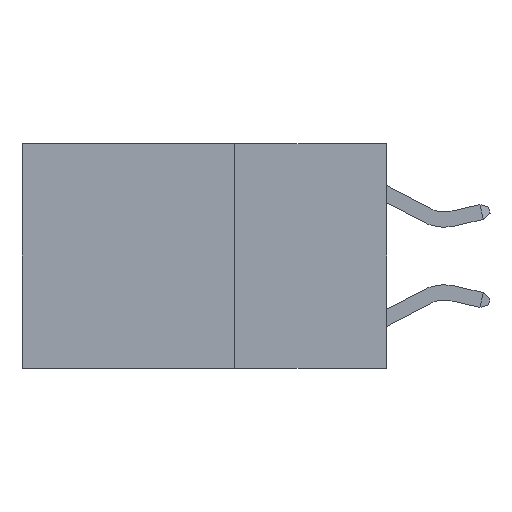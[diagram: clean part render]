
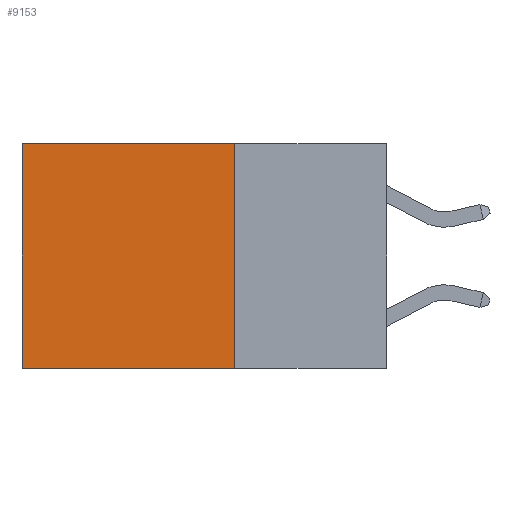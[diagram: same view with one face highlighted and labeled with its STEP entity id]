
A CAD part, left-side view. The second image highlights one B-rep face of the part: STEP entity #9153.
In plain terms, the highlighted planar face has unit normal (-1, 0, 0).
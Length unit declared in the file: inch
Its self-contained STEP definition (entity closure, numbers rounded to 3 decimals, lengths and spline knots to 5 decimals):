
#98 = VERTEX_POINT ( 'NONE', #7601 ) ;
#536 = VERTEX_POINT ( 'NONE', #4608 ) ;
#1321 = VECTOR ( 'NONE', #12298, 39.37008 ) ;
#1347 = ORIENTED_EDGE ( 'NONE', *, *, #11045, .T. ) ;
#2160 = ORIENTED_EDGE ( 'NONE', *, *, #5397, .F. ) ;
#2867 = VECTOR ( 'NONE', #4304, 39.37008 ) ;
#3821 = LINE ( 'NONE', #5575, #12467 ) ;
#4264 = CARTESIAN_POINT ( 'NONE',  ( 0.2625, 0.25, -0.37 ) ) ;
#4304 = DIRECTION ( 'NONE',  ( 0., 0., -1. ) ) ;
#4360 = CARTESIAN_POINT ( 'NONE',  ( 0.2625, 0.6, 0. ) ) ;
#4608 = CARTESIAN_POINT ( 'NONE',  ( 0.2625, 0.6, -0.37 ) ) ;
#4610 = AXIS2_PLACEMENT_3D ( 'NONE', #10485, #14152, #6821 ) ;
#4937 = CARTESIAN_POINT ( 'NONE',  ( 0.2625, 0.25, -0.37 ) ) ;
#5397 = EDGE_CURVE ( 'NONE', #11721, #536, #11530, .T. ) ;
#5575 = CARTESIAN_POINT ( 'NONE',  ( 0.2625, 0.25, 0. ) ) ;
#6766 = PLANE ( 'NONE',  #4610 ) ;
#6821 = DIRECTION ( 'NONE',  ( 0., 0., -1. ) ) ;
#7601 = CARTESIAN_POINT ( 'NONE',  ( 0.2625, 0.6, 0. ) ) ;
#9153 = ADVANCED_FACE ( 'NONE', ( #14058 ), #6766, .F. ) ;
#9445 = LINE ( 'NONE', #10458, #2867 ) ;
#9581 = CARTESIAN_POINT ( 'NONE',  ( 0.2625, 0.25, 0. ) ) ;
#10374 = EDGE_CURVE ( 'NONE', #10594, #11721, #9445, .T. ) ;
#10458 = CARTESIAN_POINT ( 'NONE',  ( 0.2625, 0.25, 0. ) ) ;
#10485 = CARTESIAN_POINT ( 'NONE',  ( 0.2625, 0.25, 0. ) ) ;
#10517 = LINE ( 'NONE', #4360, #13746 ) ;
#10594 = VERTEX_POINT ( 'NONE', #9581 ) ;
#11045 = EDGE_CURVE ( 'NONE', #10594, #98, #3821, .T. ) ;
#11530 = LINE ( 'NONE', #4937, #1321 ) ;
#11721 = VERTEX_POINT ( 'NONE', #4264 ) ;
#12298 = DIRECTION ( 'NONE',  ( 0., 1., 0. ) ) ;
#12467 = VECTOR ( 'NONE', #14154, 39.37008 ) ;
#12961 = DIRECTION ( 'NONE',  ( 0., 0., -1. ) ) ;
#13141 = ORIENTED_EDGE ( 'NONE', *, *, #13676, .T. ) ;
#13676 = EDGE_CURVE ( 'NONE', #98, #536, #10517, .T. ) ;
#13746 = VECTOR ( 'NONE', #12961, 39.37008 ) ;
#14058 = FACE_OUTER_BOUND ( 'NONE', #14068, .T. ) ;
#14068 = EDGE_LOOP ( 'NONE', ( #13141, #2160, #15311, #1347 ) ) ;
#14152 = DIRECTION ( 'NONE',  ( 1., 0., 0. ) ) ;
#14154 = DIRECTION ( 'NONE',  ( 0., 1., 0. ) ) ;
#15311 = ORIENTED_EDGE ( 'NONE', *, *, #10374, .F. ) ;
